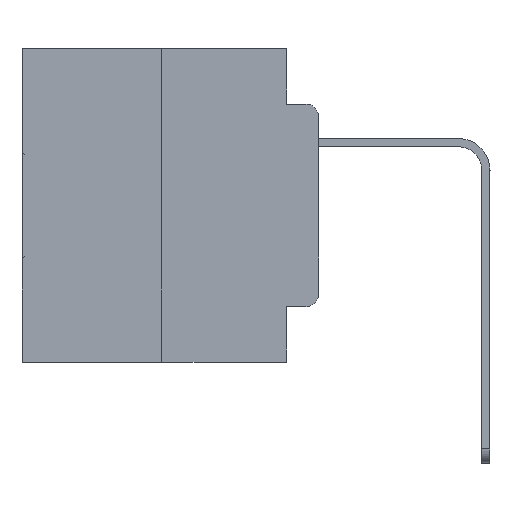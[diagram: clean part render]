
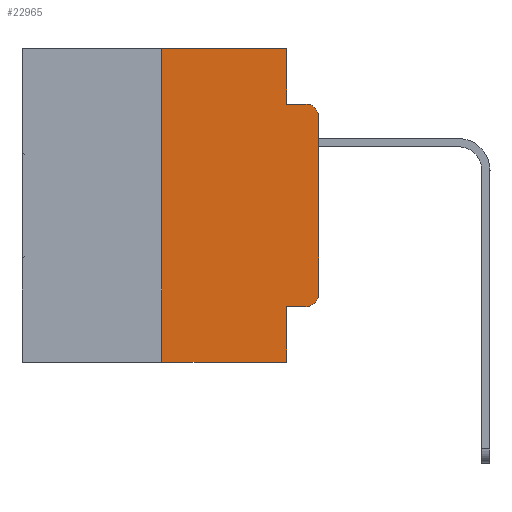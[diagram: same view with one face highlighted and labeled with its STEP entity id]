
A CAD part, left-side view. The second image highlights one B-rep face of the part: STEP entity #22965.
In plain terms, the highlighted planar face has unit normal (-1, 0, 0).
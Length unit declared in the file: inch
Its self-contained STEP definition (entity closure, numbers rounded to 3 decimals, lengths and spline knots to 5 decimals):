
#68 = VECTOR ( 'NONE', #18015, 39.37008 ) ;
#521 = VERTEX_POINT ( 'NONE', #18376 ) ;
#690 = VERTEX_POINT ( 'NONE', #23230 ) ;
#914 = VERTEX_POINT ( 'NONE', #12817 ) ;
#934 = DIRECTION ( 'NONE',  ( 0., 0., -1. ) ) ;
#985 = AXIS2_PLACEMENT_3D ( 'NONE', #10014, #28473, #14751 ) ;
#2334 = CARTESIAN_POINT ( 'NONE',  ( 0., 0.473, 0. ) ) ;
#2606 = CARTESIAN_POINT ( 'NONE',  ( 0., 0., -0.3915 ) ) ;
#2783 = DIRECTION ( 'NONE',  ( 0., 0., -1. ) ) ;
#2806 = ORIENTED_EDGE ( 'NONE', *, *, #7896, .F. ) ;
#2811 = LINE ( 'NONE', #2334, #8231 ) ;
#2938 = EDGE_CURVE ( 'NONE', #12551, #5476, #7011, .T. ) ;
#2952 = LINE ( 'NONE', #24927, #68 ) ;
#2961 = CARTESIAN_POINT ( 'NONE',  ( 0., 0.473, -0.5 ) ) ;
#3192 = EDGE_CURVE ( 'NONE', #19209, #914, #13835, .T. ) ;
#3297 = PLANE ( 'NONE',  #12349 ) ;
#3406 = CARTESIAN_POINT ( 'NONE',  ( 0., 0.051, -0.0885 ) ) ;
#3649 = LINE ( 'NONE', #14340, #11555 ) ;
#3673 = EDGE_CURVE ( 'NONE', #914, #26209, #6606, .T. ) ;
#4113 = EDGE_CURVE ( 'NONE', #28639, #521, #23175, .T. ) ;
#4205 = EDGE_CURVE ( 'NONE', #26209, #22671, #2952, .T. ) ;
#4286 = VERTEX_POINT ( 'NONE', #8098 ) ;
#5040 = ORIENTED_EDGE ( 'NONE', *, *, #3673, .T. ) ;
#5373 = EDGE_LOOP ( 'NONE', ( #23204, #20271, #15732, #16113, #2806, #14290, #14684, #22290, #25177, #5040 ) ) ;
#5476 = VERTEX_POINT ( 'NONE', #23457 ) ;
#5601 = VECTOR ( 'NONE', #2783, 39.37008 ) ;
#6606 = CIRCLE ( 'NONE', #985, 0.02 ) ;
#6692 = CARTESIAN_POINT ( 'NONE',  ( 0., 0.25, -0.5 ) ) ;
#7011 = LINE ( 'NONE', #15792, #18208 ) ;
#7066 = DIRECTION ( 'NONE',  ( 0., 0., -1. ) ) ;
#7302 = CARTESIAN_POINT ( 'NONE',  ( 0., 0.051, -0.4115 ) ) ;
#7523 = DIRECTION ( 'NONE',  ( 1., 0., 0. ) ) ;
#7896 = EDGE_CURVE ( 'NONE', #5476, #4286, #2811, .T. ) ;
#8098 = CARTESIAN_POINT ( 'NONE',  ( 0., 0.051, 0. ) ) ;
#8231 = VECTOR ( 'NONE', #20794, 39.37008 ) ;
#9111 = VECTOR ( 'NONE', #26511, 39.37008 ) ;
#9920 = DIRECTION ( 'NONE',  ( 0., -1., 0. ) ) ;
#10014 = CARTESIAN_POINT ( 'NONE',  ( 0., 0.02, -0.3915 ) ) ;
#10146 = CARTESIAN_POINT ( 'NONE',  ( 0., 0.473, 0. ) ) ;
#10236 = EDGE_CURVE ( 'NONE', #19209, #690, #18583, .T. ) ;
#11230 = DIRECTION ( 'NONE',  ( 0., 0., 1. ) ) ;
#11555 = VECTOR ( 'NONE', #934, 39.37008 ) ;
#11753 = CARTESIAN_POINT ( 'NONE',  ( 0., 0.051, 0. ) ) ;
#12093 = CARTESIAN_POINT ( 'NONE',  ( 0., 0., -0.1085 ) ) ;
#12349 = AXIS2_PLACEMENT_3D ( 'NONE', #10146, #7523, #14586 ) ;
#12551 = VERTEX_POINT ( 'NONE', #6692 ) ;
#12817 = CARTESIAN_POINT ( 'NONE',  ( 0., 0.02, -0.4115 ) ) ;
#12931 = DIRECTION ( 'NONE',  ( 0., -1., 0. ) ) ;
#13835 = LINE ( 'NONE', #26758, #25775 ) ;
#14290 = ORIENTED_EDGE ( 'NONE', *, *, #2938, .F. ) ;
#14340 = CARTESIAN_POINT ( 'NONE',  ( 0., 0.051, 0. ) ) ;
#14586 = DIRECTION ( 'NONE',  ( 0., 0., -1. ) ) ;
#14684 = ORIENTED_EDGE ( 'NONE', *, *, #28530, .T. ) ;
#14751 = DIRECTION ( 'NONE',  ( 0., 0., -1. ) ) ;
#14946 = VECTOR ( 'NONE', #9920, 39.37008 ) ;
#15507 = EDGE_CURVE ( 'NONE', #4286, #28639, #3649, .T. ) ;
#15732 = ORIENTED_EDGE ( 'NONE', *, *, #4113, .F. ) ;
#15792 = CARTESIAN_POINT ( 'NONE',  ( 0., 0.25, 0. ) ) ;
#16113 = ORIENTED_EDGE ( 'NONE', *, *, #15507, .F. ) ;
#16150 = DIRECTION ( 'NONE',  ( -1., 0., 0. ) ) ;
#17831 = CIRCLE ( 'NONE', #20050, 0.02 ) ;
#18015 = DIRECTION ( 'NONE',  ( 0., 0., 1. ) ) ;
#18208 = VECTOR ( 'NONE', #11230, 39.37008 ) ;
#18376 = CARTESIAN_POINT ( 'NONE',  ( 0., 0.02, -0.0885 ) ) ;
#18583 = LINE ( 'NONE', #11753, #5601 ) ;
#19209 = VERTEX_POINT ( 'NONE', #7302 ) ;
#20050 = AXIS2_PLACEMENT_3D ( 'NONE', #25351, #16150, #7066 ) ;
#20232 = FACE_OUTER_BOUND ( 'NONE', #5373, .T. ) ;
#20271 = ORIENTED_EDGE ( 'NONE', *, *, #20326, .T. ) ;
#20326 = EDGE_CURVE ( 'NONE', #22671, #521, #17831, .T. ) ;
#20794 = DIRECTION ( 'NONE',  ( 0., -1., 0. ) ) ;
#21076 = LINE ( 'NONE', #2961, #14946 ) ;
#22290 = ORIENTED_EDGE ( 'NONE', *, *, #10236, .F. ) ;
#22671 = VERTEX_POINT ( 'NONE', #12093 ) ;
#22965 = ADVANCED_FACE ( 'NONE', ( #20232 ), #3297, .F. ) ;
#23175 = LINE ( 'NONE', #3406, #9111 ) ;
#23204 = ORIENTED_EDGE ( 'NONE', *, *, #4205, .T. ) ;
#23230 = CARTESIAN_POINT ( 'NONE',  ( 0., 0.051, -0.5 ) ) ;
#23457 = CARTESIAN_POINT ( 'NONE',  ( 0., 0.25, 0. ) ) ;
#24927 = CARTESIAN_POINT ( 'NONE',  ( 0., 0., 0. ) ) ;
#25177 = ORIENTED_EDGE ( 'NONE', *, *, #3192, .T. ) ;
#25351 = CARTESIAN_POINT ( 'NONE',  ( 0., 0.02, -0.1085 ) ) ;
#25775 = VECTOR ( 'NONE', #12931, 39.37008 ) ;
#26209 = VERTEX_POINT ( 'NONE', #2606 ) ;
#26511 = DIRECTION ( 'NONE',  ( 0., -1., 0. ) ) ;
#26758 = CARTESIAN_POINT ( 'NONE',  ( 0., 0.051, -0.4115 ) ) ;
#28180 = CARTESIAN_POINT ( 'NONE',  ( 0., 0.051, -0.0885 ) ) ;
#28473 = DIRECTION ( 'NONE',  ( -1., 0., 0. ) ) ;
#28530 = EDGE_CURVE ( 'NONE', #12551, #690, #21076, .T. ) ;
#28639 = VERTEX_POINT ( 'NONE', #28180 ) ;
